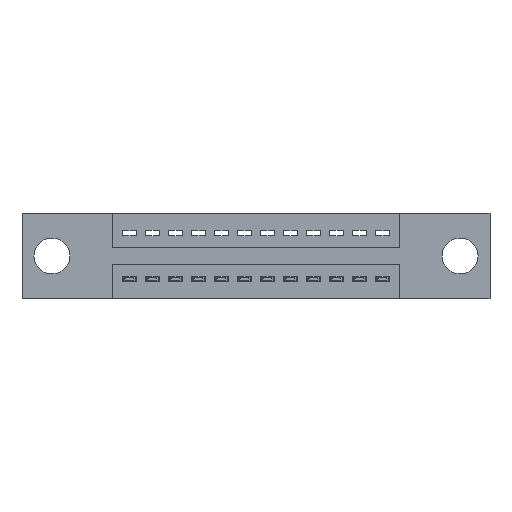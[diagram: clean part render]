
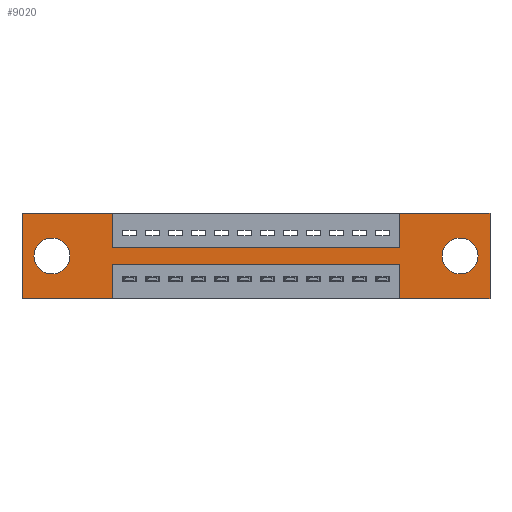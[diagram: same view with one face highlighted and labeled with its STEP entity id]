
A CAD part, front view. The second image highlights one B-rep face of the part: STEP entity #9020.
In plain terms, the highlighted planar face has unit normal (0, -1, 0).
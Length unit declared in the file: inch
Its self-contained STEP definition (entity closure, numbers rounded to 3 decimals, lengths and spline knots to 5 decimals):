
#3 = CIRCLE ( 'NONE', #418, 0.078 ) ;
#143 = DIRECTION ( 'NONE',  ( 0., 0., -1. ) ) ;
#340 = LINE ( 'NONE', #5294, #796 ) ;
#403 = AXIS2_PLACEMENT_3D ( 'NONE', #3575, #10672, #2709 ) ;
#418 = AXIS2_PLACEMENT_3D ( 'NONE', #10273, #4500, #11475 ) ;
#506 = DIRECTION ( 'NONE',  ( 0., 0., 1. ) ) ;
#560 = CARTESIAN_POINT ( 'NONE',  ( 0.3925, 0., -0.37 ) ) ;
#796 = VECTOR ( 'NONE', #11352, 39.37008 ) ;
#877 = LINE ( 'NONE', #7564, #4010 ) ;
#1347 = VECTOR ( 'NONE', #8207, 39.37008 ) ;
#1390 = CARTESIAN_POINT ( 'NONE',  ( 0.3925, 0., -0.15 ) ) ;
#1429 = CARTESIAN_POINT ( 'NONE',  ( 0.3925, 0., -0.22 ) ) ;
#1590 = CIRCLE ( 'NONE', #403, 0.078 ) ;
#1788 = LINE ( 'NONE', #560, #4439 ) ;
#1802 = EDGE_CURVE ( 'NONE', #10556, #2305, #6672, .T. ) ;
#1916 = VECTOR ( 'NONE', #10351, 39.37008 ) ;
#1918 = FACE_BOUND ( 'NONE', #8284, .T. ) ;
#1934 = ORIENTED_EDGE ( 'NONE', *, *, #6755, .T. ) ;
#1981 = CARTESIAN_POINT ( 'NONE',  ( 1.6425, 0., -0.37 ) ) ;
#2305 = VERTEX_POINT ( 'NONE', #1429 ) ;
#2511 = EDGE_CURVE ( 'NONE', #5343, #8179, #877, .T. ) ;
#2618 = CARTESIAN_POINT ( 'NONE',  ( 0.3925, 0., 0. ) ) ;
#2647 = CIRCLE ( 'NONE', #7310, 0.078 ) ;
#2700 = VECTOR ( 'NONE', #5615, 39.37008 ) ;
#2709 = DIRECTION ( 'NONE',  ( 0., 0., -1. ) ) ;
#2801 = CARTESIAN_POINT ( 'NONE',  ( 1.905, 0., -0.263 ) ) ;
#2853 = LINE ( 'NONE', #1390, #1916 ) ;
#3167 = VERTEX_POINT ( 'NONE', #5524 ) ;
#3174 = PLANE ( 'NONE',  #8252 ) ;
#3218 = ORIENTED_EDGE ( 'NONE', *, *, #10134, .F. ) ;
#3219 = EDGE_LOOP ( 'NONE', ( #12367, #5882, #10171, #12787, #3387, #3218, #5192, #4958, #8028, #4087, #11784, #9572 ) ) ;
#3359 = VERTEX_POINT ( 'NONE', #10430 ) ;
#3387 = ORIENTED_EDGE ( 'NONE', *, *, #7453, .F. ) ;
#3397 = CARTESIAN_POINT ( 'NONE',  ( 2.035, 0., 0. ) ) ;
#3452 = LINE ( 'NONE', #5598, #10938 ) ;
#3489 = EDGE_CURVE ( 'NONE', #2305, #11033, #1788, .T. ) ;
#3556 = CARTESIAN_POINT ( 'NONE',  ( 0.3925, 0., -0.22 ) ) ;
#3575 = CARTESIAN_POINT ( 'NONE',  ( 1.905, 0., -0.185 ) ) ;
#3839 = VERTEX_POINT ( 'NONE', #7656 ) ;
#4010 = VECTOR ( 'NONE', #8426, 39.37008 ) ;
#4087 = ORIENTED_EDGE ( 'NONE', *, *, #6260, .F. ) ;
#4137 = CARTESIAN_POINT ( 'NONE',  ( 0.3925, 0., -0.37 ) ) ;
#4164 = CARTESIAN_POINT ( 'NONE',  ( 0., 0., -0.37 ) ) ;
#4342 = CARTESIAN_POINT ( 'NONE',  ( 0.13, 0., -0.263 ) ) ;
#4346 = VECTOR ( 'NONE', #12717, 39.37008 ) ;
#4439 = VECTOR ( 'NONE', #6435, 39.37008 ) ;
#4450 = EDGE_CURVE ( 'NONE', #10507, #9361, #2853, .T. ) ;
#4500 = DIRECTION ( 'NONE',  ( 0., 1., 0. ) ) ;
#4550 = VERTEX_POINT ( 'NONE', #3397 ) ;
#4555 = CARTESIAN_POINT ( 'NONE',  ( 1.905, 0., -0.185 ) ) ;
#4610 = DIRECTION ( 'NONE',  ( -1., 0., 0. ) ) ;
#4661 = LINE ( 'NONE', #2618, #4346 ) ;
#4662 = EDGE_CURVE ( 'NONE', #3167, #11886, #9852, .T. ) ;
#4945 = LINE ( 'NONE', #4164, #1347 ) ;
#4958 = ORIENTED_EDGE ( 'NONE', *, *, #4450, .F. ) ;
#5066 = EDGE_CURVE ( 'NONE', #3839, #8661, #1590, .T. ) ;
#5100 = DIRECTION ( 'NONE',  ( 0., -1., 0. ) ) ;
#5182 = CARTESIAN_POINT ( 'NONE',  ( 2.035, 0., -0.37 ) ) ;
#5192 = ORIENTED_EDGE ( 'NONE', *, *, #8878, .F. ) ;
#5274 = VECTOR ( 'NONE', #12166, 39.37008 ) ;
#5294 = CARTESIAN_POINT ( 'NONE',  ( 0., 0., 0. ) ) ;
#5326 = CARTESIAN_POINT ( 'NONE',  ( 0.13, 0., -0.185 ) ) ;
#5343 = VERTEX_POINT ( 'NONE', #5182 ) ;
#5464 = ORIENTED_EDGE ( 'NONE', *, *, #6751, .T. ) ;
#5524 = CARTESIAN_POINT ( 'NONE',  ( 0., 0., -0.37 ) ) ;
#5583 = VECTOR ( 'NONE', #6915, 39.37008 ) ;
#5598 = CARTESIAN_POINT ( 'NONE',  ( 0., 0., 0. ) ) ;
#5615 = DIRECTION ( 'NONE',  ( 0., 0., 1. ) ) ;
#5623 = CARTESIAN_POINT ( 'NONE',  ( 1.6425, 0., -0.22 ) ) ;
#5655 = FACE_BOUND ( 'NONE', #9513, .T. ) ;
#5767 = CARTESIAN_POINT ( 'NONE',  ( 0.3925, 0., 0. ) ) ;
#5882 = ORIENTED_EDGE ( 'NONE', *, *, #1802, .F. ) ;
#6115 = LINE ( 'NONE', #8327, #11108 ) ;
#6260 = EDGE_CURVE ( 'NONE', #11886, #9670, #340, .T. ) ;
#6339 = DIRECTION ( 'NONE',  ( 0., 1., 0. ) ) ;
#6435 = DIRECTION ( 'NONE',  ( 0., 0., -1. ) ) ;
#6582 = CIRCLE ( 'NONE', #8676, 0.078 ) ;
#6598 = DIRECTION ( 'NONE',  ( 1., 0., 0. ) ) ;
#6672 = LINE ( 'NONE', #3556, #12288 ) ;
#6751 = EDGE_CURVE ( 'NONE', #12843, #12705, #3, .T. ) ;
#6755 = EDGE_CURVE ( 'NONE', #12705, #12843, #2647, .T. ) ;
#6848 = ORIENTED_EDGE ( 'NONE', *, *, #9990, .T. ) ;
#6915 = DIRECTION ( 'NONE',  ( 0., 0., 1. ) ) ;
#6979 = LINE ( 'NONE', #1981, #5583 ) ;
#7151 = CARTESIAN_POINT ( 'NONE',  ( 1.6425, 0., -0.15 ) ) ;
#7161 = CARTESIAN_POINT ( 'NONE',  ( 0.13, 0., -0.107 ) ) ;
#7296 = ORIENTED_EDGE ( 'NONE', *, *, #5066, .T. ) ;
#7310 = AXIS2_PLACEMENT_3D ( 'NONE', #5326, #6339, #506 ) ;
#7357 = CARTESIAN_POINT ( 'NONE',  ( 0.3925, 0., -0.15 ) ) ;
#7453 = EDGE_CURVE ( 'NONE', #4550, #5343, #9791, .T. ) ;
#7509 = DIRECTION ( 'NONE',  ( 0., 1., 0. ) ) ;
#7564 = CARTESIAN_POINT ( 'NONE',  ( 0., 0., -0.37 ) ) ;
#7656 = CARTESIAN_POINT ( 'NONE',  ( 1.905, 0., -0.107 ) ) ;
#8028 = ORIENTED_EDGE ( 'NONE', *, *, #11433, .F. ) ;
#8100 = CARTESIAN_POINT ( 'NONE',  ( 2.035, 0., 0. ) ) ;
#8133 = CARTESIAN_POINT ( 'NONE',  ( 0., 0., -0.37 ) ) ;
#8179 = VERTEX_POINT ( 'NONE', #12745 ) ;
#8207 = DIRECTION ( 'NONE',  ( -1., 0., 0. ) ) ;
#8252 = AXIS2_PLACEMENT_3D ( 'NONE', #8133, #5100, #143 ) ;
#8284 = EDGE_LOOP ( 'NONE', ( #7296, #6848 ) ) ;
#8327 = CARTESIAN_POINT ( 'NONE',  ( 1.6425, 0., 0. ) ) ;
#8426 = DIRECTION ( 'NONE',  ( -1., 0., 0. ) ) ;
#8661 = VERTEX_POINT ( 'NONE', #2801 ) ;
#8676 = AXIS2_PLACEMENT_3D ( 'NONE', #4555, #7509, #10409 ) ;
#8878 = EDGE_CURVE ( 'NONE', #9361, #3359, #6115, .T. ) ;
#9020 = ADVANCED_FACE ( 'NONE', ( #1918, #5655, #11902 ), #3174, .T. ) ;
#9361 = VERTEX_POINT ( 'NONE', #7151 ) ;
#9513 = EDGE_LOOP ( 'NONE', ( #1934, #5464 ) ) ;
#9572 = ORIENTED_EDGE ( 'NONE', *, *, #12758, .F. ) ;
#9670 = VERTEX_POINT ( 'NONE', #5767 ) ;
#9791 = LINE ( 'NONE', #8100, #5274 ) ;
#9852 = LINE ( 'NONE', #10741, #2700 ) ;
#9990 = EDGE_CURVE ( 'NONE', #8661, #3839, #6582, .T. ) ;
#10134 = EDGE_CURVE ( 'NONE', #3359, #4550, #3452, .T. ) ;
#10171 = ORIENTED_EDGE ( 'NONE', *, *, #12230, .F. ) ;
#10273 = CARTESIAN_POINT ( 'NONE',  ( 0.13, 0., -0.185 ) ) ;
#10351 = DIRECTION ( 'NONE',  ( 1., 0., 0. ) ) ;
#10409 = DIRECTION ( 'NONE',  ( 0., 0., -1. ) ) ;
#10430 = CARTESIAN_POINT ( 'NONE',  ( 1.6425, 0., 0. ) ) ;
#10507 = VERTEX_POINT ( 'NONE', #7357 ) ;
#10556 = VERTEX_POINT ( 'NONE', #5623 ) ;
#10672 = DIRECTION ( 'NONE',  ( 0., 1., 0. ) ) ;
#10741 = CARTESIAN_POINT ( 'NONE',  ( 0., 0., 0. ) ) ;
#10938 = VECTOR ( 'NONE', #6598, 39.37008 ) ;
#11033 = VERTEX_POINT ( 'NONE', #4137 ) ;
#11108 = VECTOR ( 'NONE', #11335, 39.37008 ) ;
#11335 = DIRECTION ( 'NONE',  ( 0., 0., 1. ) ) ;
#11352 = DIRECTION ( 'NONE',  ( 1., 0., 0. ) ) ;
#11433 = EDGE_CURVE ( 'NONE', #9670, #10507, #4661, .T. ) ;
#11475 = DIRECTION ( 'NONE',  ( 0., 0., 1. ) ) ;
#11784 = ORIENTED_EDGE ( 'NONE', *, *, #4662, .F. ) ;
#11886 = VERTEX_POINT ( 'NONE', #12269 ) ;
#11902 = FACE_OUTER_BOUND ( 'NONE', #3219, .T. ) ;
#12166 = DIRECTION ( 'NONE',  ( 0., 0., -1. ) ) ;
#12230 = EDGE_CURVE ( 'NONE', #8179, #10556, #6979, .T. ) ;
#12269 = CARTESIAN_POINT ( 'NONE',  ( 0., 0., 0. ) ) ;
#12288 = VECTOR ( 'NONE', #4610, 39.37008 ) ;
#12367 = ORIENTED_EDGE ( 'NONE', *, *, #3489, .F. ) ;
#12705 = VERTEX_POINT ( 'NONE', #7161 ) ;
#12717 = DIRECTION ( 'NONE',  ( 0., 0., -1. ) ) ;
#12745 = CARTESIAN_POINT ( 'NONE',  ( 1.6425, 0., -0.37 ) ) ;
#12758 = EDGE_CURVE ( 'NONE', #11033, #3167, #4945, .T. ) ;
#12787 = ORIENTED_EDGE ( 'NONE', *, *, #2511, .F. ) ;
#12843 = VERTEX_POINT ( 'NONE', #4342 ) ;
